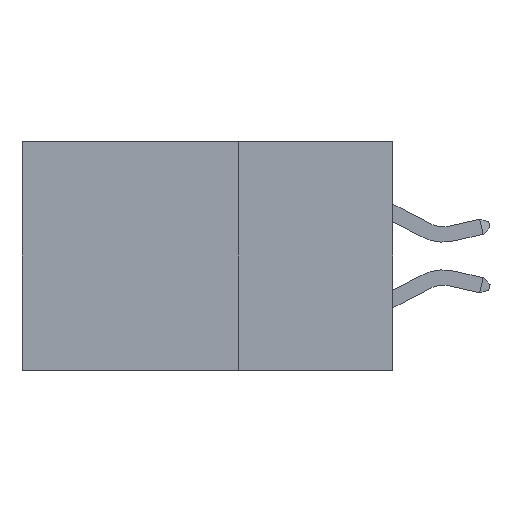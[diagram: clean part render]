
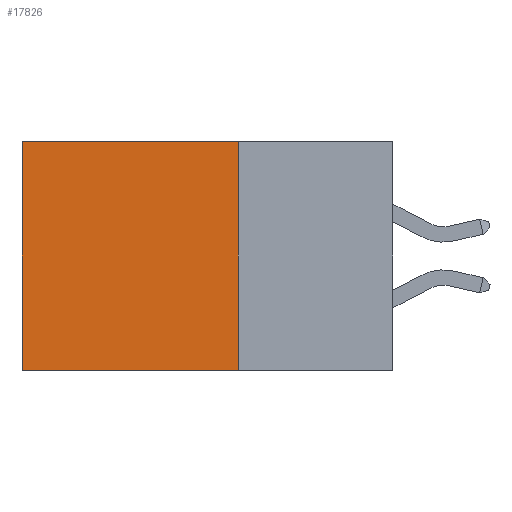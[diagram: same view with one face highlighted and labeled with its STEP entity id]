
A CAD part, left-side view. The second image highlights one B-rep face of the part: STEP entity #17826.
In plain terms, the highlighted planar face has unit normal (-1, 0, 0).
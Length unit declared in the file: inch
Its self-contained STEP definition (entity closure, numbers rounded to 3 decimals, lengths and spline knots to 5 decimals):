
#891 = VERTEX_POINT ( 'NONE', #7368 ) ;
#5358 = FACE_OUTER_BOUND ( 'NONE', #17288, .T. ) ;
#5368 = LINE ( 'NONE', #27940, #28245 ) ;
#5839 = PLANE ( 'NONE',  #29377 ) ;
#5993 = LINE ( 'NONE', #19988, #26813 ) ;
#6139 = EDGE_CURVE ( 'NONE', #30152, #10365, #6519, .T. ) ;
#6519 = LINE ( 'NONE', #17329, #8556 ) ;
#7368 = CARTESIAN_POINT ( 'NONE',  ( 0.2875, 0.25, -0.37 ) ) ;
#8556 = VECTOR ( 'NONE', #11727, 39.37008 ) ;
#10218 = ORIENTED_EDGE ( 'NONE', *, *, #6139, .T. ) ;
#10365 = VERTEX_POINT ( 'NONE', #12236 ) ;
#11397 = ORIENTED_EDGE ( 'NONE', *, *, #20950, .F. ) ;
#11727 = DIRECTION ( 'NONE',  ( 0., 0., -1. ) ) ;
#12236 = CARTESIAN_POINT ( 'NONE',  ( 0.2875, 0.6, -0.37 ) ) ;
#13248 = CARTESIAN_POINT ( 'NONE',  ( 0.2875, 0.6, 0. ) ) ;
#14769 = ORIENTED_EDGE ( 'NONE', *, *, #16231, .T. ) ;
#15348 = VERTEX_POINT ( 'NONE', #22793 ) ;
#15445 = ORIENTED_EDGE ( 'NONE', *, *, #29187, .F. ) ;
#16231 = EDGE_CURVE ( 'NONE', #15348, #30152, #20787, .T. ) ;
#16827 = DIRECTION ( 'NONE',  ( 0., 0., -1. ) ) ;
#17288 = EDGE_LOOP ( 'NONE', ( #10218, #11397, #15445, #14769 ) ) ;
#17329 = CARTESIAN_POINT ( 'NONE',  ( 0.2875, 0.6, 0. ) ) ;
#17483 = CARTESIAN_POINT ( 'NONE',  ( 0.2875, 0.25, 0. ) ) ;
#17826 = ADVANCED_FACE ( 'NONE', ( #5358 ), #5839, .F. ) ;
#19686 = DIRECTION ( 'NONE',  ( 0., 1., 0. ) ) ;
#19988 = CARTESIAN_POINT ( 'NONE',  ( 0.2875, 0.25, -0.37 ) ) ;
#20787 = LINE ( 'NONE', #17483, #27253 ) ;
#20950 = EDGE_CURVE ( 'NONE', #891, #10365, #5993, .T. ) ;
#22793 = CARTESIAN_POINT ( 'NONE',  ( 0.2875, 0.25, 0. ) ) ;
#24258 = CARTESIAN_POINT ( 'NONE',  ( 0.2875, 0.25, 0. ) ) ;
#25204 = DIRECTION ( 'NONE',  ( 0., 1., 0. ) ) ;
#26813 = VECTOR ( 'NONE', #25204, 39.37008 ) ;
#26939 = DIRECTION ( 'NONE',  ( 1., 0., 0. ) ) ;
#27253 = VECTOR ( 'NONE', #19686, 39.37008 ) ;
#27940 = CARTESIAN_POINT ( 'NONE',  ( 0.2875, 0.25, 0. ) ) ;
#28245 = VECTOR ( 'NONE', #30574, 39.37008 ) ;
#29187 = EDGE_CURVE ( 'NONE', #15348, #891, #5368, .T. ) ;
#29377 = AXIS2_PLACEMENT_3D ( 'NONE', #24258, #26939, #16827 ) ;
#30152 = VERTEX_POINT ( 'NONE', #13248 ) ;
#30574 = DIRECTION ( 'NONE',  ( 0., 0., -1. ) ) ;
